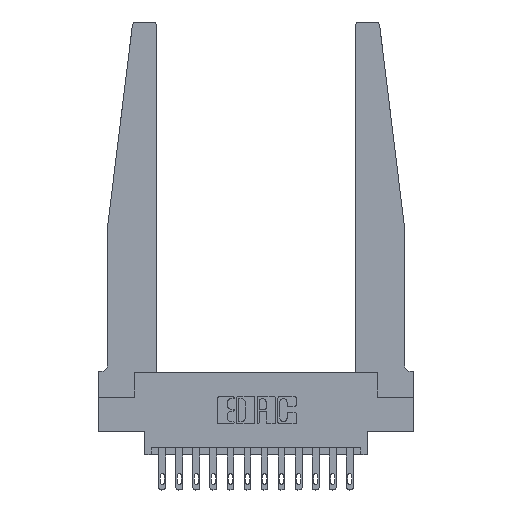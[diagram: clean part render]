
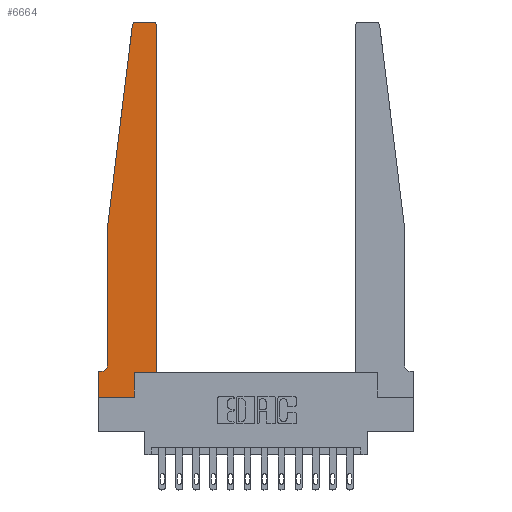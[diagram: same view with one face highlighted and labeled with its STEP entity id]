
A CAD part, top view. The second image highlights one B-rep face of the part: STEP entity #6664.
In plain terms, the highlighted planar face has unit normal (0, 0, 1).
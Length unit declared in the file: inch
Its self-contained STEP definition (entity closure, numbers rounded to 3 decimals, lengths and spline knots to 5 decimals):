
#34 = CARTESIAN_POINT ( 'NONE',  ( 0., 0.1875, 0.37 ) ) ;
#749 = DIRECTION ( 'NONE',  ( 1., 0., 0. ) ) ;
#1200 = EDGE_CURVE ( 'NONE', #12257, #9071, #7004, .T. ) ;
#1228 = ORIENTED_EDGE ( 'NONE', *, *, #14602, .T. ) ;
#1346 = VERTEX_POINT ( 'NONE', #16674 ) ;
#1633 = CARTESIAN_POINT ( 'NONE',  ( 0.395, 2.75, 0.37 ) ) ;
#1695 = LINE ( 'NONE', #13670, #8457 ) ;
#1738 = VECTOR ( 'NONE', #16619, 39.37008 ) ;
#1801 = EDGE_CURVE ( 'NONE', #7959, #3652, #10772, .T. ) ;
#1926 = VERTEX_POINT ( 'NONE', #34 ) ;
#2059 = CARTESIAN_POINT ( 'NONE',  ( 0.395, 2.72, 0.37 ) ) ;
#2080 = FACE_OUTER_BOUND ( 'NONE', #10114, .T. ) ;
#2171 = ORIENTED_EDGE ( 'NONE', *, *, #16917, .T. ) ;
#2460 = CARTESIAN_POINT ( 'NONE',  ( 0.425, 0.18, 0.37 ) ) ;
#2714 = LINE ( 'NONE', #2460, #17064 ) ;
#2743 = ORIENTED_EDGE ( 'NONE', *, *, #1200, .T. ) ;
#2921 = CARTESIAN_POINT ( 'NONE',  ( 0.065, 0.1875, 0.37 ) ) ;
#3205 = CARTESIAN_POINT ( 'NONE',  ( 0., 0.1875, 0.37 ) ) ;
#3263 = AXIS2_PLACEMENT_3D ( 'NONE', #2059, #4796, #12660 ) ;
#3340 = ORIENTED_EDGE ( 'NONE', *, *, #1801, .T. ) ;
#3374 = ORIENTED_EDGE ( 'NONE', *, *, #15191, .T. ) ;
#3430 = VERTEX_POINT ( 'NONE', #8740 ) ;
#3487 = DIRECTION ( 'NONE',  ( 0., 0., 1. ) ) ;
#3584 = EDGE_CURVE ( 'NONE', #14228, #6313, #3660, .T. ) ;
#3631 = CIRCLE ( 'NONE', #12769, 0.05 ) ;
#3652 = VERTEX_POINT ( 'NONE', #1633 ) ;
#3660 = LINE ( 'NONE', #11634, #5776 ) ;
#3688 = EDGE_CURVE ( 'NONE', #7994, #1346, #17068, .T. ) ;
#4139 = DIRECTION ( 'NONE',  ( 0., 1., 0. ) ) ;
#4174 = ORIENTED_EDGE ( 'NONE', *, *, #3584, .T. ) ;
#4219 = CARTESIAN_POINT ( 'NONE',  ( 0.2605, 0., 0.37 ) ) ;
#4345 = ORIENTED_EDGE ( 'NONE', *, *, #12296, .T. ) ;
#4602 = DIRECTION ( 'NONE',  ( 0., -1., 0. ) ) ;
#4796 = DIRECTION ( 'NONE',  ( 0., 0., 1. ) ) ;
#4850 = VERTEX_POINT ( 'NONE', #7476 ) ;
#5134 = ORIENTED_EDGE ( 'NONE', *, *, #3688, .T. ) ;
#5257 = CARTESIAN_POINT ( 'NONE',  ( 0.27653, 2.75, 0.37 ) ) ;
#5661 = CARTESIAN_POINT ( 'NONE',  ( 0.25, 2.75, 0.37 ) ) ;
#5749 = LINE ( 'NONE', #5661, #6610 ) ;
#5776 = VECTOR ( 'NONE', #10419, 39.37008 ) ;
#6313 = VERTEX_POINT ( 'NONE', #10489 ) ;
#6452 = DIRECTION ( 'NONE',  ( 0., 0., -1. ) ) ;
#6610 = VECTOR ( 'NONE', #10920, 39.37008 ) ;
#6630 = EDGE_CURVE ( 'NONE', #1346, #4850, #9957, .T. ) ;
#6664 = ADVANCED_FACE ( 'NONE', ( #2080 ), #16739, .T. ) ;
#6719 = DIRECTION ( 'NONE',  ( -1., 0., 0. ) ) ;
#6749 = AXIS2_PLACEMENT_3D ( 'NONE', #3205, #3487, #7412 ) ;
#7004 = LINE ( 'NONE', #12281, #11576 ) ;
#7165 = EDGE_CURVE ( 'NONE', #1926, #12257, #1695, .T. ) ;
#7412 = DIRECTION ( 'NONE',  ( 1., 0., 0. ) ) ;
#7476 = CARTESIAN_POINT ( 'NONE',  ( 0.065, 1.25, 0.37 ) ) ;
#7584 = CARTESIAN_POINT ( 'NONE',  ( 0.2605, 0.18, 0.37 ) ) ;
#7959 = VERTEX_POINT ( 'NONE', #9317 ) ;
#7994 = VERTEX_POINT ( 'NONE', #5257 ) ;
#8102 = ORIENTED_EDGE ( 'NONE', *, *, #13920, .T. ) ;
#8457 = VECTOR ( 'NONE', #13463, 39.37008 ) ;
#8740 = CARTESIAN_POINT ( 'NONE',  ( 0.015, 0.1875, 0.37 ) ) ;
#9071 = VERTEX_POINT ( 'NONE', #4219 ) ;
#9317 = CARTESIAN_POINT ( 'NONE',  ( 0.425, 2.72, 0.37 ) ) ;
#9787 = CARTESIAN_POINT ( 'NONE',  ( 0., 0., 0.37 ) ) ;
#9891 = DIRECTION ( 'NONE',  ( 1., 0., 0. ) ) ;
#9957 = LINE ( 'NONE', #12628, #1738 ) ;
#10114 = EDGE_LOOP ( 'NONE', ( #2171, #5134, #10284, #1228, #13164, #3374, #12343, #2743, #8102, #4174, #4345, #3340 ) ) ;
#10185 = LINE ( 'NONE', #7584, #15527 ) ;
#10284 = ORIENTED_EDGE ( 'NONE', *, *, #6630, .T. ) ;
#10419 = DIRECTION ( 'NONE',  ( 1., 0., 0. ) ) ;
#10489 = CARTESIAN_POINT ( 'NONE',  ( 0.425, 0.18, 0.37 ) ) ;
#10677 = DIRECTION ( 'NONE',  ( -1., 0., 0. ) ) ;
#10772 = CIRCLE ( 'NONE', #3263, 0.03 ) ;
#10920 = DIRECTION ( 'NONE',  ( -1., 0., 0. ) ) ;
#11576 = VECTOR ( 'NONE', #749, 39.37008 ) ;
#11634 = CARTESIAN_POINT ( 'NONE',  ( 0.425, 0.18, 0.37 ) ) ;
#11972 = CARTESIAN_POINT ( 'NONE',  ( 0.065, 0.2375, 0.37 ) ) ;
#12257 = VERTEX_POINT ( 'NONE', #9787 ) ;
#12281 = CARTESIAN_POINT ( 'NONE',  ( 0., 0., 0.37 ) ) ;
#12296 = EDGE_CURVE ( 'NONE', #6313, #7959, #2714, .T. ) ;
#12343 = ORIENTED_EDGE ( 'NONE', *, *, #7165, .T. ) ;
#12383 = AXIS2_PLACEMENT_3D ( 'NONE', #16554, #14913, #9891 ) ;
#12628 = CARTESIAN_POINT ( 'NONE',  ( 0.065, 1.25, 0.37 ) ) ;
#12660 = DIRECTION ( 'NONE',  ( 1., 0., 0. ) ) ;
#12730 = CARTESIAN_POINT ( 'NONE',  ( 0.2605, 0.18, 0.37 ) ) ;
#12769 = AXIS2_PLACEMENT_3D ( 'NONE', #14512, #6452, #6719 ) ;
#13164 = ORIENTED_EDGE ( 'NONE', *, *, #14004, .T. ) ;
#13428 = LINE ( 'NONE', #2921, #17098 ) ;
#13463 = DIRECTION ( 'NONE',  ( 0., -1., 0. ) ) ;
#13670 = CARTESIAN_POINT ( 'NONE',  ( 0., 0., 0.37 ) ) ;
#13920 = EDGE_CURVE ( 'NONE', #9071, #14228, #10185, .T. ) ;
#14004 = EDGE_CURVE ( 'NONE', #17081, #3430, #3631, .T. ) ;
#14228 = VERTEX_POINT ( 'NONE', #12730 ) ;
#14512 = CARTESIAN_POINT ( 'NONE',  ( 0.015, 0.2375, 0.37 ) ) ;
#14602 = EDGE_CURVE ( 'NONE', #4850, #17081, #15243, .T. ) ;
#14913 = DIRECTION ( 'NONE',  ( 0., 0., 1. ) ) ;
#15191 = EDGE_CURVE ( 'NONE', #3430, #1926, #13428, .T. ) ;
#15243 = LINE ( 'NONE', #16369, #15547 ) ;
#15527 = VECTOR ( 'NONE', #15540, 39.37008 ) ;
#15540 = DIRECTION ( 'NONE',  ( 0., 1., 0. ) ) ;
#15547 = VECTOR ( 'NONE', #4602, 39.37008 ) ;
#16369 = CARTESIAN_POINT ( 'NONE',  ( 0.065, 1.25, 0.37 ) ) ;
#16554 = CARTESIAN_POINT ( 'NONE',  ( 0.27653, 2.72, 0.37 ) ) ;
#16619 = DIRECTION ( 'NONE',  ( -0.122, -0.992, 0. ) ) ;
#16674 = CARTESIAN_POINT ( 'NONE',  ( 0.24675, 2.72367, 0.37 ) ) ;
#16739 = PLANE ( 'NONE',  #6749 ) ;
#16917 = EDGE_CURVE ( 'NONE', #3652, #7994, #5749, .T. ) ;
#17064 = VECTOR ( 'NONE', #4139, 39.37008 ) ;
#17068 = CIRCLE ( 'NONE', #12383, 0.03 ) ;
#17081 = VERTEX_POINT ( 'NONE', #11972 ) ;
#17098 = VECTOR ( 'NONE', #10677, 39.37008 ) ;
